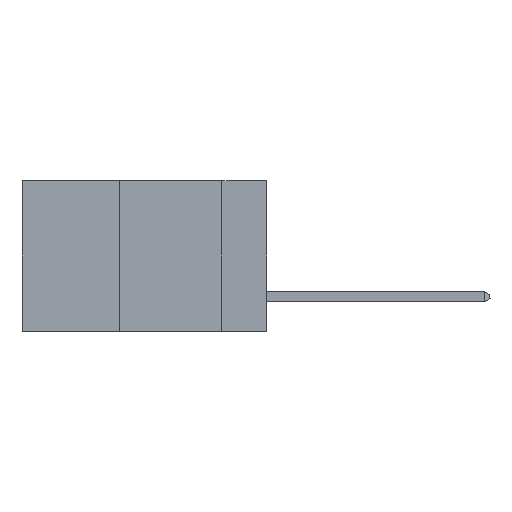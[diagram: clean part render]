
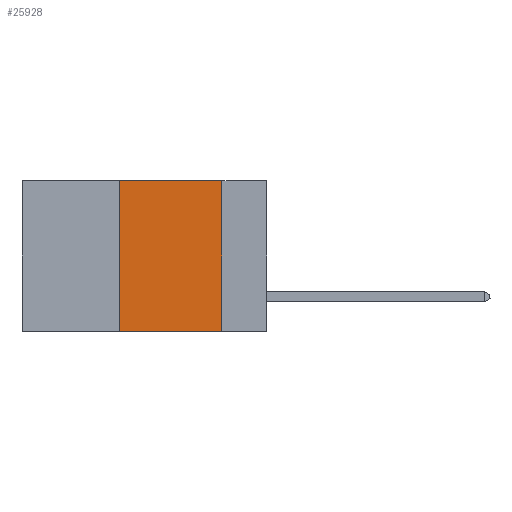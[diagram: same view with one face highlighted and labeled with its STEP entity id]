
A CAD part, left-side view. The second image highlights one B-rep face of the part: STEP entity #25928.
In plain terms, the highlighted planar face has unit normal (-1, 0, 0).
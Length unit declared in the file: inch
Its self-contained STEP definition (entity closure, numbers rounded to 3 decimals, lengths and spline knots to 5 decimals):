
#542 = PLANE ( 'NONE',  #33608 ) ;
#1581 = CARTESIAN_POINT ( 'NONE',  ( 0., 0.6, 0. ) ) ;
#4009 = CARTESIAN_POINT ( 'NONE',  ( 0., 0.11, 0. ) ) ;
#5672 = DIRECTION ( 'NONE',  ( 0., -1., 0. ) ) ;
#8090 = ORIENTED_EDGE ( 'NONE', *, *, #38457, .F. ) ;
#8536 = DIRECTION ( 'NONE',  ( 0., 0., -1. ) ) ;
#9351 = LINE ( 'NONE', #10370, #43280 ) ;
#10018 = VECTOR ( 'NONE', #5672, 39.37008 ) ;
#10370 = CARTESIAN_POINT ( 'NONE',  ( 0., 0.6, -0.37 ) ) ;
#11959 = FACE_OUTER_BOUND ( 'NONE', #35404, .T. ) ;
#12205 = EDGE_CURVE ( 'NONE', #44422, #31892, #9351, .T. ) ;
#13668 = CARTESIAN_POINT ( 'NONE',  ( 0., 0.36, -0.37 ) ) ;
#17681 = LINE ( 'NONE', #4009, #37763 ) ;
#18597 = LINE ( 'NONE', #21526, #40422 ) ;
#19341 = ORIENTED_EDGE ( 'NONE', *, *, #12205, .T. ) ;
#21526 = CARTESIAN_POINT ( 'NONE',  ( 0., 0.36, 0. ) ) ;
#22211 = DIRECTION ( 'NONE',  ( 0., -1., 0. ) ) ;
#22463 = ORIENTED_EDGE ( 'NONE', *, *, #26083, .F. ) ;
#25928 = ADVANCED_FACE ( 'NONE', ( #11959 ), #542, .F. ) ;
#26083 = EDGE_CURVE ( 'NONE', #44422, #28516, #18597, .T. ) ;
#27662 = CARTESIAN_POINT ( 'NONE',  ( 0., 0.11, -0.37 ) ) ;
#28516 = VERTEX_POINT ( 'NONE', #48562 ) ;
#30165 = EDGE_CURVE ( 'NONE', #38945, #31892, #17681, .T. ) ;
#31892 = VERTEX_POINT ( 'NONE', #27662 ) ;
#32890 = DIRECTION ( 'NONE',  ( 0., 0., 1. ) ) ;
#33608 = AXIS2_PLACEMENT_3D ( 'NONE', #43279, #35175, #8536 ) ;
#35175 = DIRECTION ( 'NONE',  ( 1., 0., 0. ) ) ;
#35404 = EDGE_LOOP ( 'NONE', ( #48869, #8090, #22463, #19341 ) ) ;
#37763 = VECTOR ( 'NONE', #39465, 39.37008 ) ;
#38457 = EDGE_CURVE ( 'NONE', #28516, #38945, #40936, .T. ) ;
#38945 = VERTEX_POINT ( 'NONE', #47979 ) ;
#39465 = DIRECTION ( 'NONE',  ( 0., 0., -1. ) ) ;
#40422 = VECTOR ( 'NONE', #32890, 39.37008 ) ;
#40936 = LINE ( 'NONE', #1581, #10018 ) ;
#43279 = CARTESIAN_POINT ( 'NONE',  ( 0., 0.6, 0. ) ) ;
#43280 = VECTOR ( 'NONE', #22211, 39.37008 ) ;
#44422 = VERTEX_POINT ( 'NONE', #13668 ) ;
#47979 = CARTESIAN_POINT ( 'NONE',  ( 0., 0.11, 0. ) ) ;
#48562 = CARTESIAN_POINT ( 'NONE',  ( 0., 0.36, 0. ) ) ;
#48869 = ORIENTED_EDGE ( 'NONE', *, *, #30165, .F. ) ;
